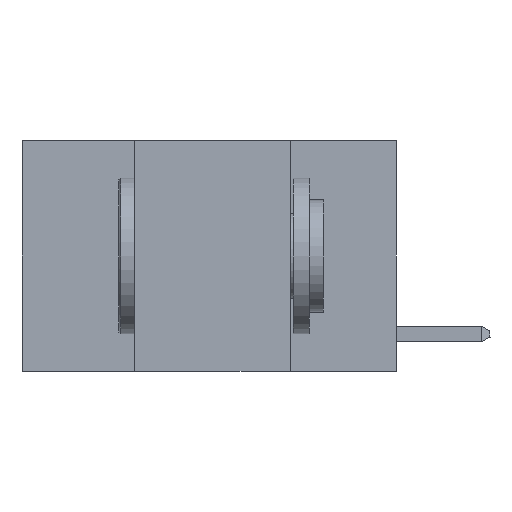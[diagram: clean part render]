
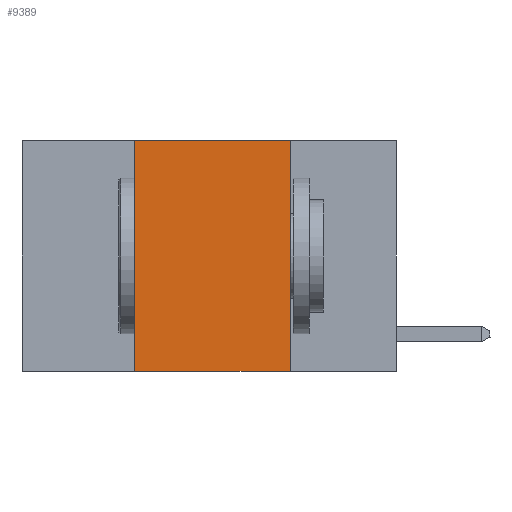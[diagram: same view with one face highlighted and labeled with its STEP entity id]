
A CAD part, left-side view. The second image highlights one B-rep face of the part: STEP entity #9389.
In plain terms, the highlighted planar face has unit normal (-1, 0, 0).
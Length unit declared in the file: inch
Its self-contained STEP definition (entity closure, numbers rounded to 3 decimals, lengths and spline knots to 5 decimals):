
#555 = AXIS2_PLACEMENT_3D ( 'NONE', #9137, #8066, #8256 ) ;
#1641 = EDGE_CURVE ( 'NONE', #4687, #3740, #7519, .T. ) ;
#1681 = PLANE ( 'NONE',  #555 ) ;
#1812 = VECTOR ( 'NONE', #11204, 39.37008 ) ;
#2145 = ORIENTED_EDGE ( 'NONE', *, *, #10544, .T. ) ;
#2187 = DIRECTION ( 'NONE',  ( 0., 0., -1. ) ) ;
#2337 = CARTESIAN_POINT ( 'NONE',  ( 0., 0.42, 0. ) ) ;
#2377 = ORIENTED_EDGE ( 'NONE', *, *, #3146, .F. ) ;
#2836 = CARTESIAN_POINT ( 'NONE',  ( 0., 0.42, -0.37 ) ) ;
#2845 = ORIENTED_EDGE ( 'NONE', *, *, #1641, .F. ) ;
#2897 = EDGE_CURVE ( 'NONE', #8553, #4687, #3906, .T. ) ;
#3146 = EDGE_CURVE ( 'NONE', #3740, #8631, #8670, .T. ) ;
#3740 = VERTEX_POINT ( 'NONE', #7830 ) ;
#3906 = LINE ( 'NONE', #5712, #1812 ) ;
#4338 = CARTESIAN_POINT ( 'NONE',  ( 0., 0.6, -0.37 ) ) ;
#4687 = VERTEX_POINT ( 'NONE', #2337 ) ;
#5101 = CARTESIAN_POINT ( 'NONE',  ( 0., 0.17, 0. ) ) ;
#5418 = FACE_OUTER_BOUND ( 'NONE', #6524, .T. ) ;
#5712 = CARTESIAN_POINT ( 'NONE',  ( 0., 0.42, 0. ) ) ;
#6417 = VECTOR ( 'NONE', #2187, 39.37008 ) ;
#6503 = DIRECTION ( 'NONE',  ( 0., -1., 0. ) ) ;
#6524 = EDGE_LOOP ( 'NONE', ( #2377, #2845, #7127, #2145 ) ) ;
#7127 = ORIENTED_EDGE ( 'NONE', *, *, #2897, .F. ) ;
#7407 = VECTOR ( 'NONE', #8021, 39.37008 ) ;
#7519 = LINE ( 'NONE', #9191, #10350 ) ;
#7830 = CARTESIAN_POINT ( 'NONE',  ( 0., 0.17, 0. ) ) ;
#7964 = LINE ( 'NONE', #4338, #7407 ) ;
#8021 = DIRECTION ( 'NONE',  ( 0., -1., 0. ) ) ;
#8066 = DIRECTION ( 'NONE',  ( 1., 0., 0. ) ) ;
#8256 = DIRECTION ( 'NONE',  ( 0., 0., -1. ) ) ;
#8553 = VERTEX_POINT ( 'NONE', #2836 ) ;
#8631 = VERTEX_POINT ( 'NONE', #9581 ) ;
#8670 = LINE ( 'NONE', #5101, #6417 ) ;
#9137 = CARTESIAN_POINT ( 'NONE',  ( 0., 0.6, 0. ) ) ;
#9191 = CARTESIAN_POINT ( 'NONE',  ( 0., 0.6, 0. ) ) ;
#9389 = ADVANCED_FACE ( 'NONE', ( #5418 ), #1681, .F. ) ;
#9581 = CARTESIAN_POINT ( 'NONE',  ( 0., 0.17, -0.37 ) ) ;
#10350 = VECTOR ( 'NONE', #6503, 39.37008 ) ;
#10544 = EDGE_CURVE ( 'NONE', #8553, #8631, #7964, .T. ) ;
#11204 = DIRECTION ( 'NONE',  ( 0., 0., 1. ) ) ;
